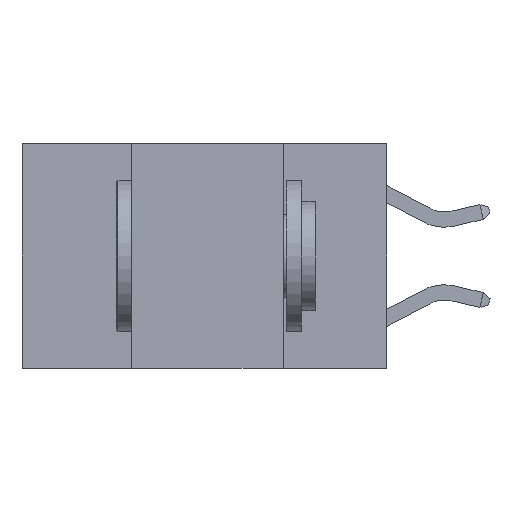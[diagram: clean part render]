
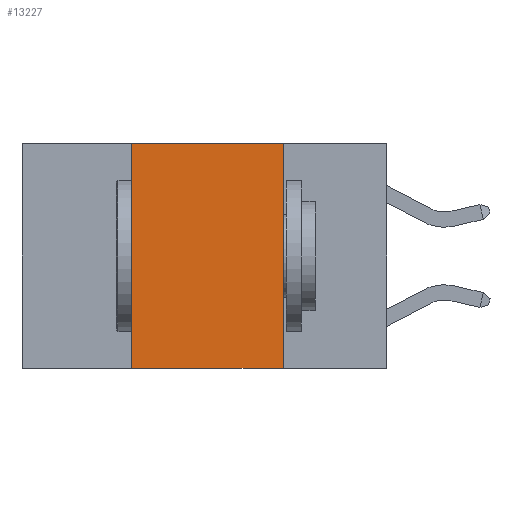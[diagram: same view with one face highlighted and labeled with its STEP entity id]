
A CAD part, left-side view. The second image highlights one B-rep face of the part: STEP entity #13227.
In plain terms, the highlighted planar face has unit normal (-1, 0, 0).
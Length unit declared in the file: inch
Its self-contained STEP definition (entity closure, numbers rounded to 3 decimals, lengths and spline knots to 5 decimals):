
#1475 = EDGE_LOOP ( 'NONE', ( #6134, #18485, #15306, #28256 ) ) ;
#2295 = CARTESIAN_POINT ( 'NONE',  ( 0., 0.42, 0. ) ) ;
#2758 = LINE ( 'NONE', #9612, #14514 ) ;
#2888 = VECTOR ( 'NONE', #10347, 39.37008 ) ;
#3215 = EDGE_CURVE ( 'NONE', #13781, #24750, #2758, .T. ) ;
#3630 = LINE ( 'NONE', #14923, #2888 ) ;
#5280 = PLANE ( 'NONE',  #26333 ) ;
#5531 = EDGE_CURVE ( 'NONE', #13781, #5733, #15815, .T. ) ;
#5733 = VERTEX_POINT ( 'NONE', #25578 ) ;
#6134 = ORIENTED_EDGE ( 'NONE', *, *, #7206, .F. ) ;
#7206 = EDGE_CURVE ( 'NONE', #13978, #5733, #3630, .T. ) ;
#7316 = DIRECTION ( 'NONE',  ( 0., -1., 0. ) ) ;
#7704 = EDGE_CURVE ( 'NONE', #24750, #13978, #20668, .T. ) ;
#8403 = VECTOR ( 'NONE', #7316, 39.37008 ) ;
#8880 = VECTOR ( 'NONE', #17985, 39.37008 ) ;
#9612 = CARTESIAN_POINT ( 'NONE',  ( 0., 0.42, 0. ) ) ;
#10046 = DIRECTION ( 'NONE',  ( 1., 0., 0. ) ) ;
#10347 = DIRECTION ( 'NONE',  ( 0., 0., -1. ) ) ;
#12075 = DIRECTION ( 'NONE',  ( 0., 0., 1. ) ) ;
#12081 = CARTESIAN_POINT ( 'NONE',  ( 0., 0.42, -0.37 ) ) ;
#12684 = CARTESIAN_POINT ( 'NONE',  ( 0., 0.17, 0. ) ) ;
#13227 = ADVANCED_FACE ( 'NONE', ( #18189 ), #5280, .F. ) ;
#13781 = VERTEX_POINT ( 'NONE', #12081 ) ;
#13978 = VERTEX_POINT ( 'NONE', #12684 ) ;
#14514 = VECTOR ( 'NONE', #12075, 39.37008 ) ;
#14923 = CARTESIAN_POINT ( 'NONE',  ( 0., 0.17, 0. ) ) ;
#15306 = ORIENTED_EDGE ( 'NONE', *, *, #3215, .F. ) ;
#15815 = LINE ( 'NONE', #29458, #8880 ) ;
#17985 = DIRECTION ( 'NONE',  ( 0., -1., 0. ) ) ;
#18189 = FACE_OUTER_BOUND ( 'NONE', #1475, .T. ) ;
#18485 = ORIENTED_EDGE ( 'NONE', *, *, #7704, .F. ) ;
#20668 = LINE ( 'NONE', #21189, #8403 ) ;
#21189 = CARTESIAN_POINT ( 'NONE',  ( 0., 0.6, 0. ) ) ;
#23915 = CARTESIAN_POINT ( 'NONE',  ( 0., 0.6, 0. ) ) ;
#24750 = VERTEX_POINT ( 'NONE', #2295 ) ;
#25578 = CARTESIAN_POINT ( 'NONE',  ( 0., 0.17, -0.37 ) ) ;
#26223 = DIRECTION ( 'NONE',  ( 0., 0., -1. ) ) ;
#26333 = AXIS2_PLACEMENT_3D ( 'NONE', #23915, #10046, #26223 ) ;
#28256 = ORIENTED_EDGE ( 'NONE', *, *, #5531, .T. ) ;
#29458 = CARTESIAN_POINT ( 'NONE',  ( 0., 0.6, -0.37 ) ) ;
